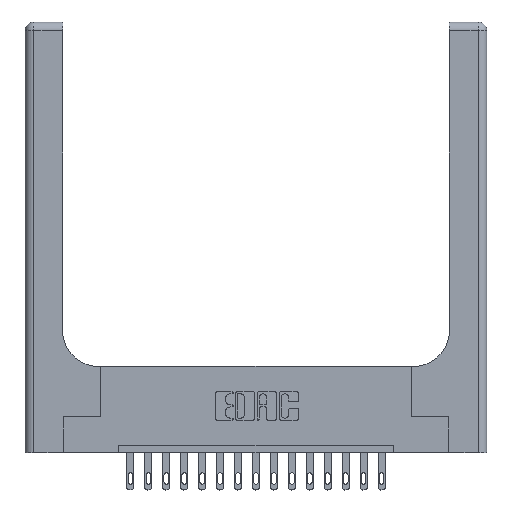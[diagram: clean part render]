
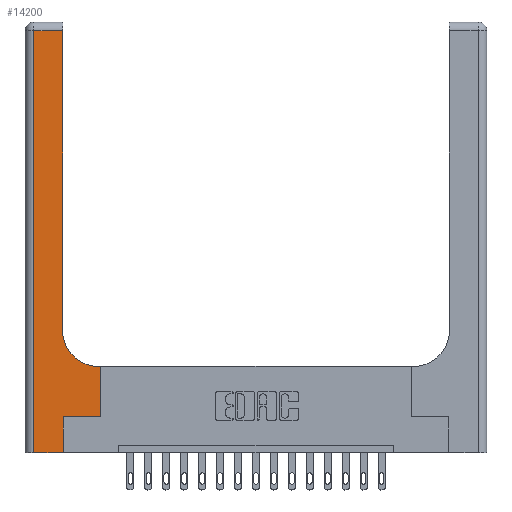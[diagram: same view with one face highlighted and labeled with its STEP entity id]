
A CAD part, top view. The second image highlights one B-rep face of the part: STEP entity #14200.
In plain terms, the highlighted planar face has unit normal (0, 0, 1).
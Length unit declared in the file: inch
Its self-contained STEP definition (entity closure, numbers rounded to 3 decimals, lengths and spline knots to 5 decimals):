
#150 = EDGE_CURVE ( 'NONE', #505, #7372, #2761, .T. ) ;
#463 = VECTOR ( 'NONE', #16845, 39.37008 ) ;
#505 = VERTEX_POINT ( 'NONE', #4040 ) ;
#542 = LINE ( 'NONE', #6232, #2398 ) ;
#652 = ORIENTED_EDGE ( 'NONE', *, *, #150, .T. ) ;
#788 = EDGE_CURVE ( 'NONE', #5498, #15019, #12142, .T. ) ;
#1495 = EDGE_CURVE ( 'NONE', #7714, #15217, #11893, .T. ) ;
#1748 = CARTESIAN_POINT ( 'NONE',  ( 0.265, 0., 0.37 ) ) ;
#2085 = LINE ( 'NONE', #7778, #6161 ) ;
#2320 = VECTOR ( 'NONE', #17010, 39.37008 ) ;
#2398 = VECTOR ( 'NONE', #11919, 39.37008 ) ;
#2476 = DIRECTION ( 'NONE',  ( 0., 1., 0. ) ) ;
#2609 = DIRECTION ( 'NONE',  ( 0., 0., -1. ) ) ;
#2761 = LINE ( 'NONE', #8474, #12984 ) ;
#3018 = ORIENTED_EDGE ( 'NONE', *, *, #9272, .T. ) ;
#3725 = DIRECTION ( 'NONE',  ( -1., 0., 0. ) ) ;
#3729 = DIRECTION ( 'NONE',  ( -1., 0., 0. ) ) ;
#3835 = AXIS2_PLACEMENT_3D ( 'NONE', #12332, #2609, #3729 ) ;
#3934 = VERTEX_POINT ( 'NONE', #16762 ) ;
#4040 = CARTESIAN_POINT ( 'NONE',  ( 0.06, 0., 0.37 ) ) ;
#4158 = VECTOR ( 'NONE', #12225, 39.37008 ) ;
#5041 = CARTESIAN_POINT ( 'NONE',  ( 0., 2.94, 0.37 ) ) ;
#5072 = ORIENTED_EDGE ( 'NONE', *, *, #15769, .T. ) ;
#5498 = VERTEX_POINT ( 'NONE', #12140 ) ;
#5956 = CARTESIAN_POINT ( 'NONE',  ( 0.51, 0.85, 0.37 ) ) ;
#6161 = VECTOR ( 'NONE', #13480, 39.37008 ) ;
#6232 = CARTESIAN_POINT ( 'NONE',  ( 0.26, 0.6, 0.37 ) ) ;
#6250 = LINE ( 'NONE', #6525, #4158 ) ;
#6292 = CARTESIAN_POINT ( 'NONE',  ( 0.528, 0.6, 0.37 ) ) ;
#6400 = DIRECTION ( 'NONE',  ( 0., 0., -1. ) ) ;
#6525 = CARTESIAN_POINT ( 'NONE',  ( 0.06, 3., 0.37 ) ) ;
#6537 = VECTOR ( 'NONE', #3725, 39.37008 ) ;
#6749 = CARTESIAN_POINT ( 'NONE',  ( 0.06, 2.94, 0.37 ) ) ;
#7173 = LINE ( 'NONE', #14079, #463 ) ;
#7372 = VERTEX_POINT ( 'NONE', #1748 ) ;
#7457 = LINE ( 'NONE', #13160, #2320 ) ;
#7714 = VERTEX_POINT ( 'NONE', #14143 ) ;
#7778 = CARTESIAN_POINT ( 'NONE',  ( 0.265, 0., 0.37 ) ) ;
#8474 = CARTESIAN_POINT ( 'NONE',  ( 0., 0., 0.37 ) ) ;
#8801 = ORIENTED_EDGE ( 'NONE', *, *, #13185, .T. ) ;
#8905 = CARTESIAN_POINT ( 'NONE',  ( 0.26, 0.85, 0.37 ) ) ;
#9272 = EDGE_CURVE ( 'NONE', #7372, #3934, #2085, .T. ) ;
#9606 = FACE_OUTER_BOUND ( 'NONE', #9880, .T. ) ;
#9764 = DIRECTION ( 'NONE',  ( 1., 0., 0. ) ) ;
#9828 = ORIENTED_EDGE ( 'NONE', *, *, #1495, .T. ) ;
#9880 = EDGE_LOOP ( 'NONE', ( #14324, #10895, #5072, #652, #3018, #14478, #8801, #13605, #9828 ) ) ;
#10154 = EDGE_CURVE ( 'NONE', #3934, #16047, #7173, .T. ) ;
#10895 = ORIENTED_EDGE ( 'NONE', *, *, #788, .T. ) ;
#10967 = DIRECTION ( 'NONE',  ( 1., 0., 0. ) ) ;
#11316 = AXIS2_PLACEMENT_3D ( 'NONE', #5956, #6400, #10967 ) ;
#11567 = CARTESIAN_POINT ( 'NONE',  ( 0.528, 0.25, 0.37 ) ) ;
#11893 = CIRCLE ( 'NONE', #11316, 0.25 ) ;
#11919 = DIRECTION ( 'NONE',  ( -1., 0., 0. ) ) ;
#12140 = CARTESIAN_POINT ( 'NONE',  ( 0.26, 2.94, 0.37 ) ) ;
#12142 = LINE ( 'NONE', #5041, #6537 ) ;
#12225 = DIRECTION ( 'NONE',  ( 0., -1., 0. ) ) ;
#12332 = CARTESIAN_POINT ( 'NONE',  ( 0., 3., 0.37 ) ) ;
#12984 = VECTOR ( 'NONE', #9764, 39.37008 ) ;
#13160 = CARTESIAN_POINT ( 'NONE',  ( 0.528, 0.25, 0.37 ) ) ;
#13185 = EDGE_CURVE ( 'NONE', #16047, #13674, #7457, .T. ) ;
#13408 = EDGE_CURVE ( 'NONE', #15217, #5498, #15637, .T. ) ;
#13480 = DIRECTION ( 'NONE',  ( 0., 1., 0. ) ) ;
#13605 = ORIENTED_EDGE ( 'NONE', *, *, #16223, .T. ) ;
#13674 = VERTEX_POINT ( 'NONE', #6292 ) ;
#14079 = CARTESIAN_POINT ( 'NONE',  ( 0.265, 0.25, 0.37 ) ) ;
#14143 = CARTESIAN_POINT ( 'NONE',  ( 0.51, 0.6, 0.37 ) ) ;
#14200 = ADVANCED_FACE ( 'NONE', ( #9606 ), #15117, .F. ) ;
#14324 = ORIENTED_EDGE ( 'NONE', *, *, #13408, .T. ) ;
#14478 = ORIENTED_EDGE ( 'NONE', *, *, #10154, .T. ) ;
#15019 = VERTEX_POINT ( 'NONE', #6749 ) ;
#15117 = PLANE ( 'NONE',  #3835 ) ;
#15217 = VERTEX_POINT ( 'NONE', #8905 ) ;
#15637 = LINE ( 'NONE', #16775, #17272 ) ;
#15769 = EDGE_CURVE ( 'NONE', #15019, #505, #6250, .T. ) ;
#16047 = VERTEX_POINT ( 'NONE', #11567 ) ;
#16223 = EDGE_CURVE ( 'NONE', #13674, #7714, #542, .T. ) ;
#16762 = CARTESIAN_POINT ( 'NONE',  ( 0.265, 0.25, 0.37 ) ) ;
#16775 = CARTESIAN_POINT ( 'NONE',  ( 0.26, 3., 0.37 ) ) ;
#16845 = DIRECTION ( 'NONE',  ( 1., 0., 0. ) ) ;
#17010 = DIRECTION ( 'NONE',  ( 0., 1., 0. ) ) ;
#17272 = VECTOR ( 'NONE', #2476, 39.37008 ) ;
